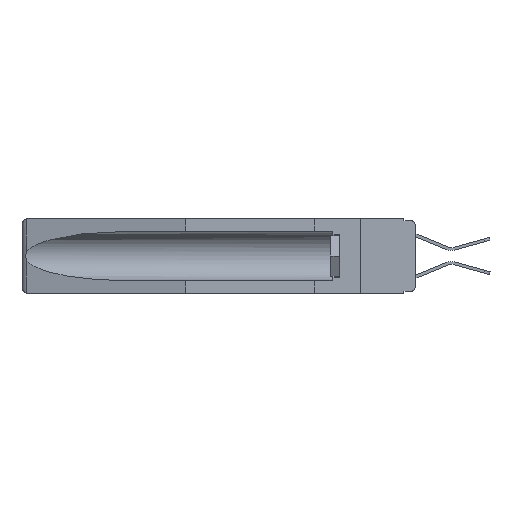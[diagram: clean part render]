
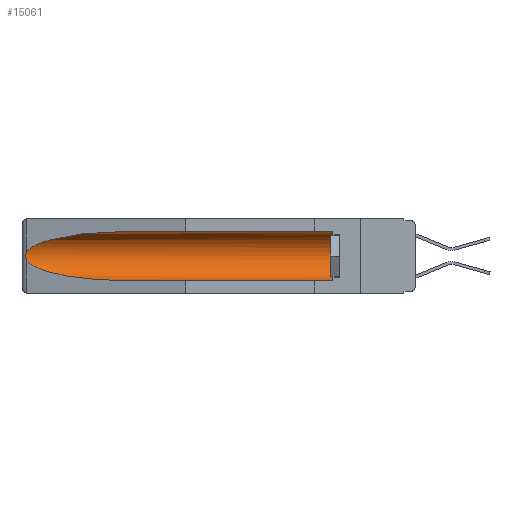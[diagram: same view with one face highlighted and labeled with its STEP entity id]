
A CAD part, left-side view. The second image highlights one B-rep face of the part: STEP entity #15061.
In plain terms, the highlighted cylindrical face has radius 2.857 mm (diameter 5.715 mm), a partial arc.
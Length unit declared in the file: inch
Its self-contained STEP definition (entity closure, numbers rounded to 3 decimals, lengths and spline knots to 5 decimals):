
#618 = CARTESIAN_POINT ( 'NONE',  ( 0.155, -0.30754, -0.1715 ) ) ;
#811 = EDGE_CURVE ( 'NONE', #5042, #17765, #2942, .T. ) ;
#939 = CARTESIAN_POINT ( 'NONE',  ( 0.155, 0.126, -0.059 ) ) ;
#1092 = LINE ( 'NONE', #2227, #9925 ) ;
#1343 = CIRCLE ( 'NONE', #15463, 0.1125 ) ;
#1425 = CYLINDRICAL_SURFACE ( 'NONE', #14809, 0.1125 ) ;
#2210 = ORIENTED_EDGE ( 'NONE', *, *, #8861, .T. ) ;
#2227 = CARTESIAN_POINT ( 'NONE',  ( 0.155, -0.30754, -0.059 ) ) ;
#2942 = LINE ( 'NONE', #7418, #19198 ) ;
#2951 = CARTESIAN_POINT ( 'NONE',  ( 0.26537, 1.52718, -0.14972 ) ) ;
#3240 = CARTESIAN_POINT ( 'NONE',  ( 0.25451, 1.48313, -0.24835 ) ) ;
#3397 = DIRECTION ( 'NONE',  ( 0., 0., 1. ) ) ;
#3587 = ORIENTED_EDGE ( 'NONE', *, *, #12783, .T. ) ;
#4596 = CARTESIAN_POINT ( 'NONE',  ( 0.2675, 1.53308, -0.17534 ) ) ;
#4754 = CARTESIAN_POINT ( 'NONE',  ( 0.155, 0.126, -0.284 ) ) ;
#4873 = CARTESIAN_POINT ( 'NONE',  ( 0.155, 0.126, -0.1715 ) ) ;
#5042 = VERTEX_POINT ( 'NONE', #4754 ) ;
#5156 = DIRECTION ( 'NONE',  ( 0., 1., 0. ) ) ;
#5965 = CARTESIAN_POINT ( 'NONE',  ( 0.26655, 1.53094, -0.18657 ) ) ;
#6156 = CARTESIAN_POINT ( 'NONE',  ( 0.2673, 1.53269, -0.17917 ) ) ;
#6370 = ORIENTED_EDGE ( 'NONE', *, *, #13407, .T. ) ;
#7356 =( BOUNDED_CURVE ( )  B_SPLINE_CURVE ( 3, ( #18261, #3240, #13045, #18620 ),
 .UNSPECIFIED., .F., .F. ) 
 B_SPLINE_CURVE_WITH_KNOTS ( ( 4, 4 ),
 ( 0.1948, 1.5708 ),
 .UNSPECIFIED. ) 
 CURVE ( )  GEOMETRIC_REPRESENTATION_ITEM ( )  RATIONAL_B_SPLINE_CURVE ( ( 1., 0.848, 0.848, 1. ) ) 
 REPRESENTATION_ITEM ( '' )  );
#7418 = CARTESIAN_POINT ( 'NONE',  ( 0.155, -0.30754, -0.284 ) ) ;
#7425 = VERTEX_POINT ( 'NONE', #7700 ) ;
#7587 = CARTESIAN_POINT ( 'NONE',  ( 0.26597, 1.5296, -0.19026 ) ) ;
#7700 = CARTESIAN_POINT ( 'NONE',  ( 0.155, 1.07973, -0.059 ) ) ;
#8051 = EDGE_CURVE ( 'NONE', #5042, #18949, #1343, .T. ) ;
#8440 = VERTEX_POINT ( 'NONE', #10148 ) ;
#8753 = ORIENTED_EDGE ( 'NONE', *, *, #8051, .T. ) ;
#8861 = EDGE_CURVE ( 'NONE', #18949, #7425, #1092, .T. ) ;
#9144 = CARTESIAN_POINT ( 'NONE',  ( 0.26537, 1.52718, -0.14972 ) ) ;
#9596 = DIRECTION ( 'NONE',  ( 0., 0., 1. ) ) ;
#9925 = VECTOR ( 'NONE', #15731, 39.37008 ) ;
#10148 = CARTESIAN_POINT ( 'NONE',  ( 0.26537, 1.52718, -0.19328 ) ) ;
#10411 = CARTESIAN_POINT ( 'NONE',  ( 0.2673, 1.5327, -0.16383 ) ) ;
#10880 = DIRECTION ( 'NONE',  ( 0., -1., 0. ) ) ;
#12175 = CARTESIAN_POINT ( 'NONE',  ( 0.155, 1.07973, -0.284 ) ) ;
#12783 = EDGE_CURVE ( 'NONE', #8440, #17765, #7356, .T. ) ;
#12848 = VERTEX_POINT ( 'NONE', #9144 ) ;
#13045 = CARTESIAN_POINT ( 'NONE',  ( 0.21114, 1.30732, -0.284 ) ) ;
#13257 = DIRECTION ( 'NONE',  ( 0., 1., 0. ) ) ;
#13368 = CARTESIAN_POINT ( 'NONE',  ( 0.155, 1.07973, -0.059 ) ) ;
#13407 = EDGE_CURVE ( 'NONE', #7425, #12848, #17741, .T. ) ;
#14809 = AXIS2_PLACEMENT_3D ( 'NONE', #618, #5156, #9596 ) ;
#14894 = CARTESIAN_POINT ( 'NONE',  ( 0.2675, 1.53308, -0.16763 ) ) ;
#15061 = ADVANCED_FACE ( 'NONE', ( #18622 ), #1425, .F. ) ;
#15449 = EDGE_LOOP ( 'NONE', ( #6370, #18530, #3587, #15999, #8753, #2210 ) ) ;
#15463 = AXIS2_PLACEMENT_3D ( 'NONE', #4873, #10880, #3397 ) ;
#15731 = DIRECTION ( 'NONE',  ( 0., 1., 0. ) ) ;
#15999 = ORIENTED_EDGE ( 'NONE', *, *, #811, .F. ) ;
#16197 = CARTESIAN_POINT ( 'NONE',  ( 0.21114, 1.30732, -0.059 ) ) ;
#16302 = B_SPLINE_CURVE_WITH_KNOTS ( 'NONE', 3,
 ( #18961, #19151, #17865, #10411, #14894, #4596, #6156, #5965, #7587, #16504 ),
 .UNSPECIFIED., .F., .F.,
 ( 4, 2, 2, 2, 4 ),
 ( 0., 0.00029, 0.00058, 0.00087, 0.00117 ),
 .UNSPECIFIED. ) ;
#16504 = CARTESIAN_POINT ( 'NONE',  ( 0.26537, 1.52718, -0.19328 ) ) ;
#17741 =( BOUNDED_CURVE ( )  B_SPLINE_CURVE ( 3, ( #13368, #16197, #19037, #2951 ),
 .UNSPECIFIED., .F., .F. ) 
 B_SPLINE_CURVE_WITH_KNOTS ( ( 4, 4 ),
 ( 4.71239, 6.08839 ),
 .UNSPECIFIED. ) 
 CURVE ( )  GEOMETRIC_REPRESENTATION_ITEM ( )  RATIONAL_B_SPLINE_CURVE ( ( 1., 0.848, 0.848, 1. ) ) 
 REPRESENTATION_ITEM ( '' )  );
#17765 = VERTEX_POINT ( 'NONE', #12175 ) ;
#17865 = CARTESIAN_POINT ( 'NONE',  ( 0.26654, 1.53092, -0.15636 ) ) ;
#18261 = CARTESIAN_POINT ( 'NONE',  ( 0.26537, 1.52718, -0.19328 ) ) ;
#18530 = ORIENTED_EDGE ( 'NONE', *, *, #19163, .T. ) ;
#18620 = CARTESIAN_POINT ( 'NONE',  ( 0.155, 1.07973, -0.284 ) ) ;
#18622 = FACE_OUTER_BOUND ( 'NONE', #15449, .T. ) ;
#18949 = VERTEX_POINT ( 'NONE', #939 ) ;
#18961 = CARTESIAN_POINT ( 'NONE',  ( 0.26537, 1.52718, -0.14972 ) ) ;
#19037 = CARTESIAN_POINT ( 'NONE',  ( 0.25451, 1.48313, -0.09465 ) ) ;
#19151 = CARTESIAN_POINT ( 'NONE',  ( 0.26597, 1.52961, -0.15275 ) ) ;
#19163 = EDGE_CURVE ( 'NONE', #12848, #8440, #16302, .T. ) ;
#19198 = VECTOR ( 'NONE', #13257, 39.37008 ) ;
